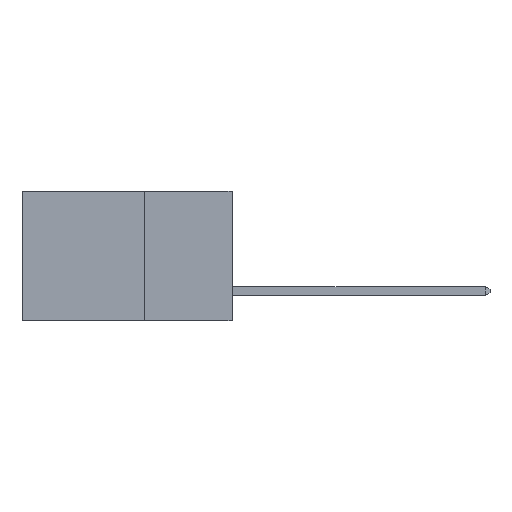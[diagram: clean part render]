
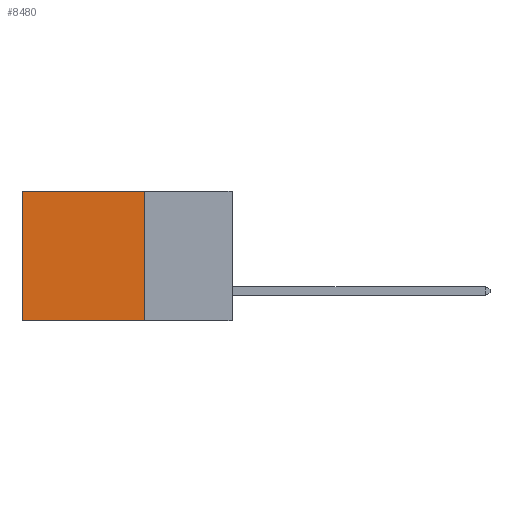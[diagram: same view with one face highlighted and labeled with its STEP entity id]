
A CAD part, left-side view. The second image highlights one B-rep face of the part: STEP entity #8480.
In plain terms, the highlighted planar face has unit normal (-1, 0, 0).
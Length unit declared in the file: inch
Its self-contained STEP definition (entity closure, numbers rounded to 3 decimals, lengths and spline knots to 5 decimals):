
#152 = CARTESIAN_POINT ( 'NONE',  ( 0.2875, 0.25, -0.37 ) ) ;
#522 = VECTOR ( 'NONE', #10536, 39.37008 ) ;
#534 = EDGE_CURVE ( 'NONE', #10235, #12742, #10830, .T. ) ;
#1874 = FACE_OUTER_BOUND ( 'NONE', #8326, .T. ) ;
#2530 = VECTOR ( 'NONE', #14102, 39.37008 ) ;
#2768 = CARTESIAN_POINT ( 'NONE',  ( 0.2875, 0.6, -0.37 ) ) ;
#3013 = LINE ( 'NONE', #4262, #2530 ) ;
#3291 = ORIENTED_EDGE ( 'NONE', *, *, #14975, .T. ) ;
#3396 = AXIS2_PLACEMENT_3D ( 'NONE', #11457, #8741, #18184 ) ;
#3923 = CARTESIAN_POINT ( 'NONE',  ( 0.2875, 0.25, 0. ) ) ;
#4059 = EDGE_CURVE ( 'NONE', #11896, #12742, #4159, .T. ) ;
#4159 = LINE ( 'NONE', #152, #522 ) ;
#4262 = CARTESIAN_POINT ( 'NONE',  ( 0.2875, 0.25, 0. ) ) ;
#5767 = VECTOR ( 'NONE', #15633, 39.37008 ) ;
#6575 = VERTEX_POINT ( 'NONE', #3923 ) ;
#7037 = CARTESIAN_POINT ( 'NONE',  ( 0.2875, 0.6, 0. ) ) ;
#7071 = DIRECTION ( 'NONE',  ( 0., 0., -1. ) ) ;
#7470 = CARTESIAN_POINT ( 'NONE',  ( 0.2875, 0.25, 0. ) ) ;
#8326 = EDGE_LOOP ( 'NONE', ( #16933, #12757, #13741, #3291 ) ) ;
#8480 = ADVANCED_FACE ( 'NONE', ( #1874 ), #15500, .F. ) ;
#8741 = DIRECTION ( 'NONE',  ( 1., 0., 0. ) ) ;
#10235 = VERTEX_POINT ( 'NONE', #14032 ) ;
#10536 = DIRECTION ( 'NONE',  ( 0., 1., 0. ) ) ;
#10830 = LINE ( 'NONE', #7037, #17557 ) ;
#11457 = CARTESIAN_POINT ( 'NONE',  ( 0.2875, 0.25, 0. ) ) ;
#11896 = VERTEX_POINT ( 'NONE', #14998 ) ;
#12196 = EDGE_CURVE ( 'NONE', #6575, #11896, #12369, .T. ) ;
#12369 = LINE ( 'NONE', #7470, #5767 ) ;
#12742 = VERTEX_POINT ( 'NONE', #2768 ) ;
#12757 = ORIENTED_EDGE ( 'NONE', *, *, #4059, .F. ) ;
#13741 = ORIENTED_EDGE ( 'NONE', *, *, #12196, .F. ) ;
#14032 = CARTESIAN_POINT ( 'NONE',  ( 0.2875, 0.6, 0. ) ) ;
#14102 = DIRECTION ( 'NONE',  ( 0., 1., 0. ) ) ;
#14975 = EDGE_CURVE ( 'NONE', #6575, #10235, #3013, .T. ) ;
#14998 = CARTESIAN_POINT ( 'NONE',  ( 0.2875, 0.25, -0.37 ) ) ;
#15500 = PLANE ( 'NONE',  #3396 ) ;
#15633 = DIRECTION ( 'NONE',  ( 0., 0., -1. ) ) ;
#16933 = ORIENTED_EDGE ( 'NONE', *, *, #534, .T. ) ;
#17557 = VECTOR ( 'NONE', #7071, 39.37008 ) ;
#18184 = DIRECTION ( 'NONE',  ( 0., 0., -1. ) ) ;
